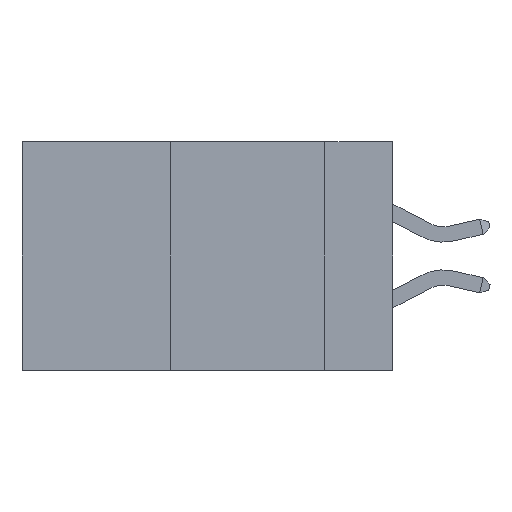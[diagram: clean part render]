
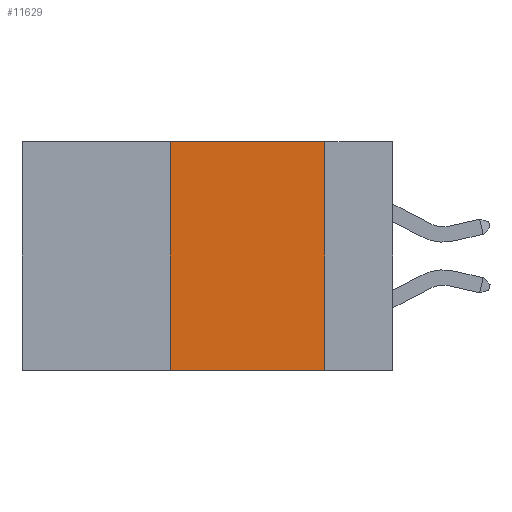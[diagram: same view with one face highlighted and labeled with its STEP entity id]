
A CAD part, left-side view. The second image highlights one B-rep face of the part: STEP entity #11629.
In plain terms, the highlighted planar face has unit normal (-1, 0, 0).
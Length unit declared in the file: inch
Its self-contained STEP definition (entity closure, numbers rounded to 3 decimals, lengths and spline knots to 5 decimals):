
#1078 = VECTOR ( 'NONE', #4434, 39.37008 ) ;
#1231 = CARTESIAN_POINT ( 'NONE',  ( 0., 0.36, 0. ) ) ;
#1383 = EDGE_CURVE ( 'NONE', #3066, #17121, #11509, .T. ) ;
#1879 = LINE ( 'NONE', #18155, #1078 ) ;
#2505 = VERTEX_POINT ( 'NONE', #4374 ) ;
#2765 = CARTESIAN_POINT ( 'NONE',  ( 0., 0.6, -0.37 ) ) ;
#3066 = VERTEX_POINT ( 'NONE', #12563 ) ;
#3426 = AXIS2_PLACEMENT_3D ( 'NONE', #4287, #19892, #21563 ) ;
#4287 = CARTESIAN_POINT ( 'NONE',  ( 0., 0.6, 0. ) ) ;
#4374 = CARTESIAN_POINT ( 'NONE',  ( 0., 0.11, -0.37 ) ) ;
#4434 = DIRECTION ( 'NONE',  ( 0., 0., -1. ) ) ;
#4660 = DIRECTION ( 'NONE',  ( 0., 0., 1. ) ) ;
#6049 = EDGE_CURVE ( 'NONE', #11846, #3066, #13412, .T. ) ;
#6701 = DIRECTION ( 'NONE',  ( 0., -1., 0. ) ) ;
#6950 = VECTOR ( 'NONE', #6701, 39.37008 ) ;
#7132 = ORIENTED_EDGE ( 'NONE', *, *, #21720, .F. ) ;
#7296 = FACE_OUTER_BOUND ( 'NONE', #14310, .T. ) ;
#7549 = ORIENTED_EDGE ( 'NONE', *, *, #15876, .T. ) ;
#7857 = PLANE ( 'NONE',  #3426 ) ;
#9666 = DIRECTION ( 'NONE',  ( 0., -1., 0. ) ) ;
#11509 = LINE ( 'NONE', #18642, #6950 ) ;
#11629 = ADVANCED_FACE ( 'NONE', ( #7296 ), #7857, .F. ) ;
#11846 = VERTEX_POINT ( 'NONE', #11973 ) ;
#11973 = CARTESIAN_POINT ( 'NONE',  ( 0., 0.36, -0.37 ) ) ;
#12058 = VECTOR ( 'NONE', #4660, 39.37008 ) ;
#12563 = CARTESIAN_POINT ( 'NONE',  ( 0., 0.36, 0. ) ) ;
#13412 = LINE ( 'NONE', #1231, #12058 ) ;
#13679 = ORIENTED_EDGE ( 'NONE', *, *, #1383, .F. ) ;
#14310 = EDGE_LOOP ( 'NONE', ( #7132, #13679, #20044, #7549 ) ) ;
#14821 = VECTOR ( 'NONE', #9666, 39.37008 ) ;
#15076 = LINE ( 'NONE', #2765, #14821 ) ;
#15876 = EDGE_CURVE ( 'NONE', #11846, #2505, #15076, .T. ) ;
#17121 = VERTEX_POINT ( 'NONE', #21562 ) ;
#18155 = CARTESIAN_POINT ( 'NONE',  ( 0., 0.11, 0. ) ) ;
#18642 = CARTESIAN_POINT ( 'NONE',  ( 0., 0.6, 0. ) ) ;
#19892 = DIRECTION ( 'NONE',  ( 1., 0., 0. ) ) ;
#20044 = ORIENTED_EDGE ( 'NONE', *, *, #6049, .F. ) ;
#21562 = CARTESIAN_POINT ( 'NONE',  ( 0., 0.11, 0. ) ) ;
#21563 = DIRECTION ( 'NONE',  ( 0., 0., -1. ) ) ;
#21720 = EDGE_CURVE ( 'NONE', #17121, #2505, #1879, .T. ) ;
